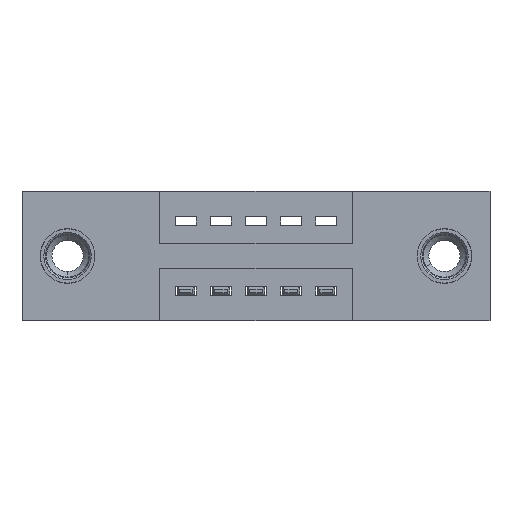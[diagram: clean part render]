
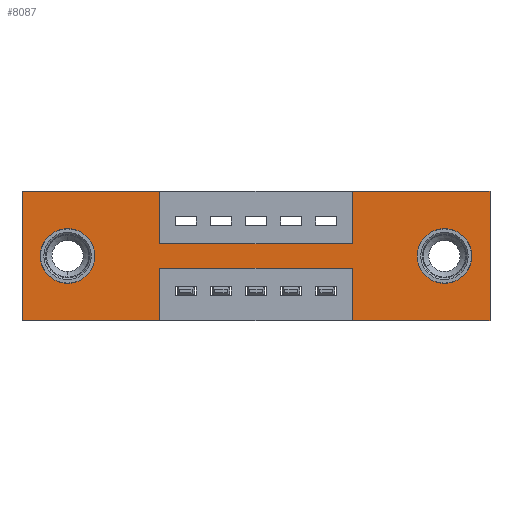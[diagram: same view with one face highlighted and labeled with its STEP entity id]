
A CAD part, front view. The second image highlights one B-rep face of the part: STEP entity #8087.
In plain terms, the highlighted planar face has unit normal (0, -1, 0).
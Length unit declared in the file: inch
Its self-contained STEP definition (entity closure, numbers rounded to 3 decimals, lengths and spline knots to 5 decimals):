
#77 = VECTOR ( 'NONE', #2733, 39.37008 ) ;
#111 = CARTESIAN_POINT ( 'NONE',  ( 0.9425, 0., -0.37 ) ) ;
#152 = CARTESIAN_POINT ( 'NONE',  ( 0.3925, 0., -0.22 ) ) ;
#168 = CARTESIAN_POINT ( 'NONE',  ( 0.13, 0., -0.263 ) ) ;
#280 = AXIS2_PLACEMENT_3D ( 'NONE', #343, #1132, #6437 ) ;
#319 = VECTOR ( 'NONE', #2254, 39.37008 ) ;
#343 = CARTESIAN_POINT ( 'NONE',  ( 0., 0., -0.37 ) ) ;
#389 = CARTESIAN_POINT ( 'NONE',  ( 0.13, 0., -0.185 ) ) ;
#546 = DIRECTION ( 'NONE',  ( 0., 0., 1. ) ) ;
#788 = CARTESIAN_POINT ( 'NONE',  ( 0.3925, 0., -0.15 ) ) ;
#814 = LINE ( 'NONE', #3706, #6818 ) ;
#924 = LINE ( 'NONE', #1343, #8463 ) ;
#928 = CARTESIAN_POINT ( 'NONE',  ( 1.205, 0., -0.263 ) ) ;
#994 = ORIENTED_EDGE ( 'NONE', *, *, #7621, .F. ) ;
#999 = CARTESIAN_POINT ( 'NONE',  ( 1.205, 0., -0.107 ) ) ;
#1034 = PLANE ( 'NONE',  #280 ) ;
#1128 = EDGE_CURVE ( 'NONE', #6360, #5245, #6248, .T. ) ;
#1132 = DIRECTION ( 'NONE',  ( 0., -1., 0. ) ) ;
#1181 = FACE_BOUND ( 'NONE', #5002, .T. ) ;
#1343 = CARTESIAN_POINT ( 'NONE',  ( 0., 0., -0.37 ) ) ;
#1364 = DIRECTION ( 'NONE',  ( 1., 0., 0. ) ) ;
#1401 = CARTESIAN_POINT ( 'NONE',  ( 0.9425, 0., 0. ) ) ;
#1571 = DIRECTION ( 'NONE',  ( 0., 0., -1. ) ) ;
#1633 = DIRECTION ( 'NONE',  ( -1., 0., 0. ) ) ;
#1635 = CARTESIAN_POINT ( 'NONE',  ( 0., 0., 0. ) ) ;
#1674 = ORIENTED_EDGE ( 'NONE', *, *, #7187, .F. ) ;
#1718 = AXIS2_PLACEMENT_3D ( 'NONE', #3422, #2788, #6451 ) ;
#1791 = ORIENTED_EDGE ( 'NONE', *, *, #3332, .F. ) ;
#1820 = EDGE_CURVE ( 'NONE', #9352, #9472, #924, .T. ) ;
#1954 = VERTEX_POINT ( 'NONE', #7592 ) ;
#2069 = DIRECTION ( 'NONE',  ( 0., 0., -1. ) ) ;
#2115 = ORIENTED_EDGE ( 'NONE', *, *, #2264, .F. ) ;
#2138 = CARTESIAN_POINT ( 'NONE',  ( 0.9425, 0., -0.15 ) ) ;
#2217 = ORIENTED_EDGE ( 'NONE', *, *, #8199, .F. ) ;
#2248 = VECTOR ( 'NONE', #4761, 39.37008 ) ;
#2254 = DIRECTION ( 'NONE',  ( 0., 0., 1. ) ) ;
#2264 = EDGE_CURVE ( 'NONE', #7708, #9352, #6554, .T. ) ;
#2294 = ORIENTED_EDGE ( 'NONE', *, *, #7516, .F. ) ;
#2319 = CARTESIAN_POINT ( 'NONE',  ( 0., 0., -0.37 ) ) ;
#2560 = LINE ( 'NONE', #4471, #319 ) ;
#2716 = FACE_BOUND ( 'NONE', #7339, .T. ) ;
#2733 = DIRECTION ( 'NONE',  ( 0., 0., -1. ) ) ;
#2788 = DIRECTION ( 'NONE',  ( 0., 1., 0. ) ) ;
#2928 = EDGE_CURVE ( 'NONE', #1954, #4629, #814, .T. ) ;
#2998 = DIRECTION ( 'NONE',  ( -1., 0., 0. ) ) ;
#3034 = EDGE_LOOP ( 'NONE', ( #2115, #2217, #4093, #994, #6030, #2294, #1791, #5085, #1674, #7176, #8261, #5633 ) ) ;
#3154 = VECTOR ( 'NONE', #4879, 39.37008 ) ;
#3332 = EDGE_CURVE ( 'NONE', #5872, #8922, #4913, .T. ) ;
#3422 = CARTESIAN_POINT ( 'NONE',  ( 0.13, 0., -0.185 ) ) ;
#3522 = CARTESIAN_POINT ( 'NONE',  ( 0., 0., -0.37 ) ) ;
#3706 = CARTESIAN_POINT ( 'NONE',  ( 1.335, 0., 0. ) ) ;
#3711 = DIRECTION ( 'NONE',  ( 0., 1., 0. ) ) ;
#3719 = VERTEX_POINT ( 'NONE', #788 ) ;
#3743 = CARTESIAN_POINT ( 'NONE',  ( 1.205, 0., -0.185 ) ) ;
#3767 = CIRCLE ( 'NONE', #6914, 0.078 ) ;
#3789 = VECTOR ( 'NONE', #1364, 39.37008 ) ;
#3912 = ORIENTED_EDGE ( 'NONE', *, *, #8771, .T. ) ;
#4093 = ORIENTED_EDGE ( 'NONE', *, *, #9535, .F. ) ;
#4362 = VECTOR ( 'NONE', #2998, 39.37008 ) ;
#4390 = VERTEX_POINT ( 'NONE', #168 ) ;
#4443 = CARTESIAN_POINT ( 'NONE',  ( 0.9425, 0., -0.22 ) ) ;
#4471 = CARTESIAN_POINT ( 'NONE',  ( 0.9425, 0., -0.37 ) ) ;
#4510 = DIRECTION ( 'NONE',  ( 0., 0., -1. ) ) ;
#4531 = EDGE_CURVE ( 'NONE', #3719, #5872, #9489, .T. ) ;
#4549 = CIRCLE ( 'NONE', #1718, 0.078 ) ;
#4615 = VECTOR ( 'NONE', #7311, 39.37008 ) ;
#4629 = VERTEX_POINT ( 'NONE', #8664 ) ;
#4661 = EDGE_CURVE ( 'NONE', #4390, #7778, #4549, .T. ) ;
#4761 = DIRECTION ( 'NONE',  ( 0., 0., 1. ) ) ;
#4769 = DIRECTION ( 'NONE',  ( 1., 0., 0. ) ) ;
#4879 = DIRECTION ( 'NONE',  ( 0., 0., 1. ) ) ;
#4885 = AXIS2_PLACEMENT_3D ( 'NONE', #8562, #5787, #2069 ) ;
#4913 = LINE ( 'NONE', #8680, #3154 ) ;
#5002 = EDGE_LOOP ( 'NONE', ( #8077, #6589 ) ) ;
#5085 = ORIENTED_EDGE ( 'NONE', *, *, #4531, .F. ) ;
#5118 = ORIENTED_EDGE ( 'NONE', *, *, #4661, .T. ) ;
#5245 = VERTEX_POINT ( 'NONE', #999 ) ;
#5272 = CARTESIAN_POINT ( 'NONE',  ( 0.3925, 0., -0.22 ) ) ;
#5481 = VERTEX_POINT ( 'NONE', #8162 ) ;
#5633 = ORIENTED_EDGE ( 'NONE', *, *, #1820, .F. ) ;
#5667 = LINE ( 'NONE', #6098, #7691 ) ;
#5787 = DIRECTION ( 'NONE',  ( 0., 1., 0. ) ) ;
#5794 = LINE ( 'NONE', #6507, #4615 ) ;
#5807 = CARTESIAN_POINT ( 'NONE',  ( 0.3925, 0., 0. ) ) ;
#5872 = VERTEX_POINT ( 'NONE', #2138 ) ;
#6030 = ORIENTED_EDGE ( 'NONE', *, *, #2928, .F. ) ;
#6035 = VECTOR ( 'NONE', #1633, 39.37008 ) ;
#6098 = CARTESIAN_POINT ( 'NONE',  ( 0.3925, 0., 0. ) ) ;
#6248 = CIRCLE ( 'NONE', #8725, 0.078 ) ;
#6360 = VERTEX_POINT ( 'NONE', #928 ) ;
#6437 = DIRECTION ( 'NONE',  ( 0., 0., -1. ) ) ;
#6451 = DIRECTION ( 'NONE',  ( 0., 0., 1. ) ) ;
#6507 = CARTESIAN_POINT ( 'NONE',  ( 0., 0., 0. ) ) ;
#6554 = LINE ( 'NONE', #8716, #77 ) ;
#6557 = EDGE_CURVE ( 'NONE', #5481, #7818, #6618, .T. ) ;
#6589 = ORIENTED_EDGE ( 'NONE', *, *, #1128, .T. ) ;
#6618 = LINE ( 'NONE', #7381, #3789 ) ;
#6627 = DIRECTION ( 'NONE',  ( -1., 0., 0. ) ) ;
#6708 = EDGE_CURVE ( 'NONE', #9472, #5481, #7913, .T. ) ;
#6709 = DIRECTION ( 'NONE',  ( 0., 1., 0. ) ) ;
#6817 = VERTEX_POINT ( 'NONE', #111 ) ;
#6818 = VECTOR ( 'NONE', #9769, 39.37008 ) ;
#6914 = AXIS2_PLACEMENT_3D ( 'NONE', #389, #6709, #546 ) ;
#7176 = ORIENTED_EDGE ( 'NONE', *, *, #6557, .F. ) ;
#7187 = EDGE_CURVE ( 'NONE', #7818, #3719, #5667, .T. ) ;
#7311 = DIRECTION ( 'NONE',  ( 1., 0., 0. ) ) ;
#7319 = FACE_OUTER_BOUND ( 'NONE', #3034, .T. ) ;
#7339 = EDGE_LOOP ( 'NONE', ( #3912, #5118 ) ) ;
#7381 = CARTESIAN_POINT ( 'NONE',  ( 0., 0., 0. ) ) ;
#7516 = EDGE_CURVE ( 'NONE', #8922, #1954, #5794, .T. ) ;
#7592 = CARTESIAN_POINT ( 'NONE',  ( 1.335, 0., 0. ) ) ;
#7621 = EDGE_CURVE ( 'NONE', #4629, #6817, #9104, .T. ) ;
#7691 = VECTOR ( 'NONE', #1571, 39.37008 ) ;
#7708 = VERTEX_POINT ( 'NONE', #152 ) ;
#7778 = VERTEX_POINT ( 'NONE', #7892 ) ;
#7811 = CARTESIAN_POINT ( 'NONE',  ( 0.3925, 0., -0.15 ) ) ;
#7818 = VERTEX_POINT ( 'NONE', #5807 ) ;
#7840 = VERTEX_POINT ( 'NONE', #4443 ) ;
#7892 = CARTESIAN_POINT ( 'NONE',  ( 0.13, 0., -0.107 ) ) ;
#7913 = LINE ( 'NONE', #1635, #2248 ) ;
#8077 = ORIENTED_EDGE ( 'NONE', *, *, #9097, .T. ) ;
#8087 = ADVANCED_FACE ( 'NONE', ( #1181, #2716, #7319 ), #1034, .T. ) ;
#8162 = CARTESIAN_POINT ( 'NONE',  ( 0., 0., 0. ) ) ;
#8199 = EDGE_CURVE ( 'NONE', #7840, #7708, #8611, .T. ) ;
#8261 = ORIENTED_EDGE ( 'NONE', *, *, #6708, .F. ) ;
#8369 = CARTESIAN_POINT ( 'NONE',  ( 0.3925, 0., -0.37 ) ) ;
#8463 = VECTOR ( 'NONE', #6627, 39.37008 ) ;
#8562 = CARTESIAN_POINT ( 'NONE',  ( 1.205, 0., -0.185 ) ) ;
#8611 = LINE ( 'NONE', #5272, #4362 ) ;
#8664 = CARTESIAN_POINT ( 'NONE',  ( 1.335, 0., -0.37 ) ) ;
#8680 = CARTESIAN_POINT ( 'NONE',  ( 0.9425, 0., 0. ) ) ;
#8696 = CIRCLE ( 'NONE', #4885, 0.078 ) ;
#8716 = CARTESIAN_POINT ( 'NONE',  ( 0.3925, 0., -0.37 ) ) ;
#8725 = AXIS2_PLACEMENT_3D ( 'NONE', #3743, #3711, #4510 ) ;
#8771 = EDGE_CURVE ( 'NONE', #7778, #4390, #3767, .T. ) ;
#8921 = VECTOR ( 'NONE', #4769, 39.37008 ) ;
#8922 = VERTEX_POINT ( 'NONE', #1401 ) ;
#9097 = EDGE_CURVE ( 'NONE', #5245, #6360, #8696, .T. ) ;
#9104 = LINE ( 'NONE', #2319, #6035 ) ;
#9352 = VERTEX_POINT ( 'NONE', #8369 ) ;
#9472 = VERTEX_POINT ( 'NONE', #3522 ) ;
#9489 = LINE ( 'NONE', #7811, #8921 ) ;
#9535 = EDGE_CURVE ( 'NONE', #6817, #7840, #2560, .T. ) ;
#9769 = DIRECTION ( 'NONE',  ( 0., 0., -1. ) ) ;
